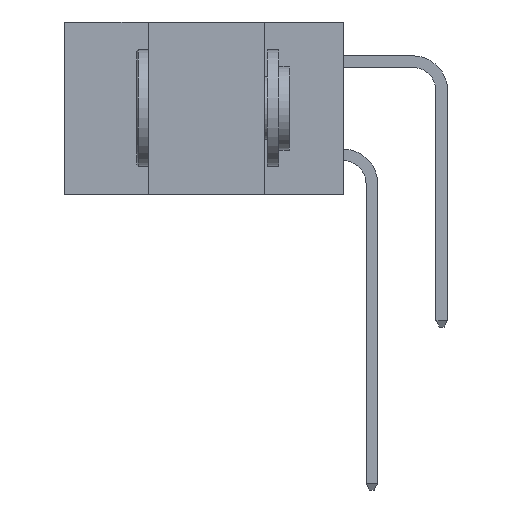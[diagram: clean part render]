
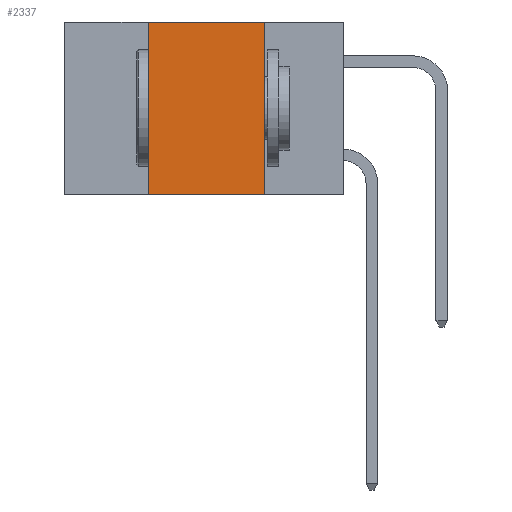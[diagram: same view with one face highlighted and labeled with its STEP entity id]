
A CAD part, left-side view. The second image highlights one B-rep face of the part: STEP entity #2337.
In plain terms, the highlighted planar face has unit normal (-1, 0, 0).
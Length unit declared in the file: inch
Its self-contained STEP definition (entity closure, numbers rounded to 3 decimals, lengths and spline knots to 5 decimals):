
#683 = CARTESIAN_POINT ( 'NONE',  ( 0., 0.42, 0. ) ) ;
#1651 = LINE ( 'NONE', #15711, #5974 ) ;
#1687 = VERTEX_POINT ( 'NONE', #12148 ) ;
#2337 = ADVANCED_FACE ( 'NONE', ( #2861 ), #3799, .F. ) ;
#2723 = VERTEX_POINT ( 'NONE', #683 ) ;
#2861 = FACE_OUTER_BOUND ( 'NONE', #27815, .T. ) ;
#3163 = VERTEX_POINT ( 'NONE', #25940 ) ;
#3250 = VECTOR ( 'NONE', #25401, 39.37008 ) ;
#3569 = LINE ( 'NONE', #6034, #15054 ) ;
#3799 = PLANE ( 'NONE',  #7649 ) ;
#4594 = LINE ( 'NONE', #5929, #3250 ) ;
#4947 = DIRECTION ( 'NONE',  ( 0., -1., 0. ) ) ;
#5929 = CARTESIAN_POINT ( 'NONE',  ( 0., 0.6, 0. ) ) ;
#5946 = DIRECTION ( 'NONE',  ( 1., 0., 0. ) ) ;
#5974 = VECTOR ( 'NONE', #4947, 39.37008 ) ;
#6034 = CARTESIAN_POINT ( 'NONE',  ( 0., 0.42, -0.37 ) ) ;
#7649 = AXIS2_PLACEMENT_3D ( 'NONE', #19008, #5946, #21159 ) ;
#8194 = EDGE_CURVE ( 'NONE', #1687, #2723, #3569, .T. ) ;
#8950 = VERTEX_POINT ( 'NONE', #14994 ) ;
#8958 = VECTOR ( 'NONE', #23135, 39.37008 ) ;
#12148 = CARTESIAN_POINT ( 'NONE',  ( 0., 0.42, -0.37 ) ) ;
#12211 = CARTESIAN_POINT ( 'NONE',  ( 0., 0.17, -0.37 ) ) ;
#14387 = ORIENTED_EDGE ( 'NONE', *, *, #17138, .T. ) ;
#14994 = CARTESIAN_POINT ( 'NONE',  ( 0., 0.17, -0.37 ) ) ;
#15054 = VECTOR ( 'NONE', #21259, 39.37008 ) ;
#15711 = CARTESIAN_POINT ( 'NONE',  ( 0., 0.6, -0.37 ) ) ;
#17138 = EDGE_CURVE ( 'NONE', #1687, #8950, #1651, .T. ) ;
#18128 = EDGE_CURVE ( 'NONE', #2723, #3163, #4594, .T. ) ;
#19008 = CARTESIAN_POINT ( 'NONE',  ( 0., 0.6, 0. ) ) ;
#19788 = ORIENTED_EDGE ( 'NONE', *, *, #8194, .F. ) ;
#20592 = LINE ( 'NONE', #12211, #8958 ) ;
#21159 = DIRECTION ( 'NONE',  ( 0., 0., -1. ) ) ;
#21259 = DIRECTION ( 'NONE',  ( 0., 0., 1. ) ) ;
#22444 = ORIENTED_EDGE ( 'NONE', *, *, #18128, .F. ) ;
#22572 = ORIENTED_EDGE ( 'NONE', *, *, #22751, .F. ) ;
#22751 = EDGE_CURVE ( 'NONE', #3163, #8950, #20592, .T. ) ;
#23135 = DIRECTION ( 'NONE',  ( 0., 0., -1. ) ) ;
#25401 = DIRECTION ( 'NONE',  ( 0., -1., 0. ) ) ;
#25940 = CARTESIAN_POINT ( 'NONE',  ( 0., 0.17, 0. ) ) ;
#27815 = EDGE_LOOP ( 'NONE', ( #22572, #22444, #19788, #14387 ) ) ;
